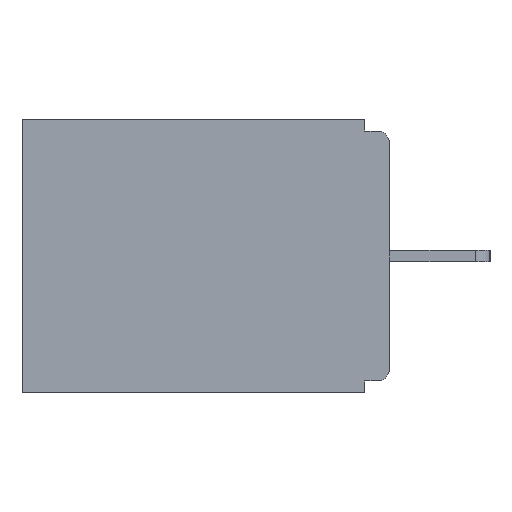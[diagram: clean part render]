
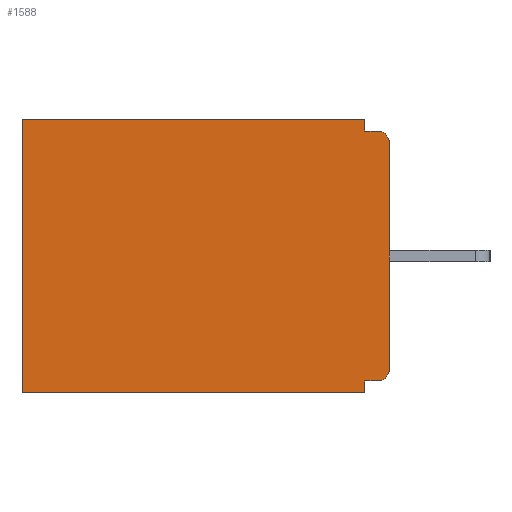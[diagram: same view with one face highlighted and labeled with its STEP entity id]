
A CAD part, left-side view. The second image highlights one B-rep face of the part: STEP entity #1588.
In plain terms, the highlighted planar face has unit normal (-1, 0, 0).
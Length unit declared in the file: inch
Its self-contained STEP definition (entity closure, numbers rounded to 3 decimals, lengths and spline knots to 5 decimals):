
#13 = VERTEX_POINT ( 'NONE', #4970 ) ;
#422 = CARTESIAN_POINT ( 'NONE',  ( 0.298, 0.031, -0.015 ) ) ;
#600 = CARTESIAN_POINT ( 'NONE',  ( 0.298, 0.015, -0.03 ) ) ;
#796 = LINE ( 'NONE', #12673, #15736 ) ;
#1186 = ORIENTED_EDGE ( 'NONE', *, *, #9808, .F. ) ;
#1255 = VECTOR ( 'NONE', #13989, 39.37008 ) ;
#1539 = EDGE_CURVE ( 'NONE', #2392, #10683, #5908, .T. ) ;
#1588 = ADVANCED_FACE ( 'NONE', ( #13958 ), #13664, .F. ) ;
#1697 = VECTOR ( 'NONE', #10648, 39.37008 ) ;
#1818 = CARTESIAN_POINT ( 'NONE',  ( 0.298, 0.46, 0. ) ) ;
#1954 = VECTOR ( 'NONE', #9693, 39.37008 ) ;
#2392 = VERTEX_POINT ( 'NONE', #10952 ) ;
#2653 = LINE ( 'NONE', #12521, #1954 ) ;
#2800 = LINE ( 'NONE', #5910, #7103 ) ;
#2859 = VERTEX_POINT ( 'NONE', #9610 ) ;
#3008 = CARTESIAN_POINT ( 'NONE',  ( 0.298, 0.031, -0.343 ) ) ;
#3226 = ORIENTED_EDGE ( 'NONE', *, *, #16742, .T. ) ;
#3445 = CARTESIAN_POINT ( 'NONE',  ( 0.298, 0., 0. ) ) ;
#3633 = DIRECTION ( 'NONE',  ( 1., 0., 0. ) ) ;
#3678 = EDGE_CURVE ( 'NONE', #2859, #18352, #16409, .T. ) ;
#3740 = EDGE_CURVE ( 'NONE', #10683, #18352, #2653, .T. ) ;
#4431 = ORIENTED_EDGE ( 'NONE', *, *, #3740, .F. ) ;
#4865 = CARTESIAN_POINT ( 'NONE',  ( 0.298, 0., -0.015 ) ) ;
#4866 = DIRECTION ( 'NONE',  ( 0., 0., -1. ) ) ;
#4970 = CARTESIAN_POINT ( 'NONE',  ( 0.298, 0., -0.03 ) ) ;
#4979 = DIRECTION ( 'NONE',  ( 0., 0., -1. ) ) ;
#5305 = VERTEX_POINT ( 'NONE', #6427 ) ;
#5325 = EDGE_CURVE ( 'NONE', #14812, #2859, #10608, .T. ) ;
#5695 = VERTEX_POINT ( 'NONE', #422 ) ;
#5908 = LINE ( 'NONE', #7524, #10994 ) ;
#5910 = CARTESIAN_POINT ( 'NONE',  ( 0.298, 0., -0.328 ) ) ;
#5939 = EDGE_CURVE ( 'NONE', #14812, #5695, #796, .T. ) ;
#6337 = DIRECTION ( 'NONE',  ( 0., 1., 0. ) ) ;
#6427 = CARTESIAN_POINT ( 'NONE',  ( 0.298, 0., -0.313 ) ) ;
#6455 = CARTESIAN_POINT ( 'NONE',  ( 0.298, 0.015, -0.015 ) ) ;
#6488 = VECTOR ( 'NONE', #14982, 39.37008 ) ;
#6786 = ORIENTED_EDGE ( 'NONE', *, *, #11349, .F. ) ;
#7095 = CARTESIAN_POINT ( 'NONE',  ( 0.298, 0.031, 0. ) ) ;
#7103 = VECTOR ( 'NONE', #14356, 39.37008 ) ;
#7524 = CARTESIAN_POINT ( 'NONE',  ( 0.298, 0.031, -0.343 ) ) ;
#7583 = ORIENTED_EDGE ( 'NONE', *, *, #3678, .T. ) ;
#7736 = DIRECTION ( 'NONE',  ( -1., 0., 0. ) ) ;
#7809 = LINE ( 'NONE', #4865, #1697 ) ;
#8090 = DIRECTION ( 'NONE',  ( 0., 0., -1. ) ) ;
#8124 = LINE ( 'NONE', #17129, #1255 ) ;
#9147 = DIRECTION ( 'NONE',  ( -1., 0., 0. ) ) ;
#9610 = CARTESIAN_POINT ( 'NONE',  ( 0.298, 0.46, 0. ) ) ;
#9693 = DIRECTION ( 'NONE',  ( 0., 1., 0. ) ) ;
#9808 = EDGE_CURVE ( 'NONE', #14503, #2392, #2800, .T. ) ;
#10076 = ORIENTED_EDGE ( 'NONE', *, *, #18541, .T. ) ;
#10523 = ORIENTED_EDGE ( 'NONE', *, *, #1539, .F. ) ;
#10608 = LINE ( 'NONE', #16571, #11460 ) ;
#10648 = DIRECTION ( 'NONE',  ( 0., -1., 0. ) ) ;
#10683 = VERTEX_POINT ( 'NONE', #3008 ) ;
#10952 = CARTESIAN_POINT ( 'NONE',  ( 0.298, 0.031, -0.328 ) ) ;
#10994 = VECTOR ( 'NONE', #13199, 39.37008 ) ;
#11256 = CIRCLE ( 'NONE', #14876, 0.015 ) ;
#11349 = EDGE_CURVE ( 'NONE', #5695, #14223, #7809, .T. ) ;
#11460 = VECTOR ( 'NONE', #6337, 39.37008 ) ;
#12340 = ORIENTED_EDGE ( 'NONE', *, *, #5939, .F. ) ;
#12401 = CIRCLE ( 'NONE', #16035, 0.015 ) ;
#12521 = CARTESIAN_POINT ( 'NONE',  ( 0.298, 0., -0.343 ) ) ;
#12673 = CARTESIAN_POINT ( 'NONE',  ( 0.298, 0.031, -0.343 ) ) ;
#13199 = DIRECTION ( 'NONE',  ( 0., 0., -1. ) ) ;
#13627 = EDGE_LOOP ( 'NONE', ( #3226, #6786, #12340, #14045, #7583, #4431, #10523, #1186, #10076, #16776 ) ) ;
#13664 = PLANE ( 'NONE',  #14324 ) ;
#13958 = FACE_OUTER_BOUND ( 'NONE', #13627, .T. ) ;
#13989 = DIRECTION ( 'NONE',  ( 0., 0., -1. ) ) ;
#14045 = ORIENTED_EDGE ( 'NONE', *, *, #5325, .T. ) ;
#14223 = VERTEX_POINT ( 'NONE', #6455 ) ;
#14324 = AXIS2_PLACEMENT_3D ( 'NONE', #3445, #3633, #8090 ) ;
#14356 = DIRECTION ( 'NONE',  ( 0., 1., 0. ) ) ;
#14503 = VERTEX_POINT ( 'NONE', #16016 ) ;
#14812 = VERTEX_POINT ( 'NONE', #7095 ) ;
#14876 = AXIS2_PLACEMENT_3D ( 'NONE', #18052, #9147, #4866 ) ;
#14982 = DIRECTION ( 'NONE',  ( 0., 0., -1. ) ) ;
#15736 = VECTOR ( 'NONE', #18466, 39.37008 ) ;
#16016 = CARTESIAN_POINT ( 'NONE',  ( 0.298, 0.015, -0.328 ) ) ;
#16035 = AXIS2_PLACEMENT_3D ( 'NONE', #600, #7736, #4979 ) ;
#16409 = LINE ( 'NONE', #1818, #6488 ) ;
#16571 = CARTESIAN_POINT ( 'NONE',  ( 0.298, 0., 0. ) ) ;
#16742 = EDGE_CURVE ( 'NONE', #13, #14223, #12401, .T. ) ;
#16776 = ORIENTED_EDGE ( 'NONE', *, *, #18282, .F. ) ;
#17129 = CARTESIAN_POINT ( 'NONE',  ( 0.298, 0., 0. ) ) ;
#17405 = CARTESIAN_POINT ( 'NONE',  ( 0.298, 0.46, -0.343 ) ) ;
#18052 = CARTESIAN_POINT ( 'NONE',  ( 0.298, 0.015, -0.313 ) ) ;
#18282 = EDGE_CURVE ( 'NONE', #13, #5305, #8124, .T. ) ;
#18352 = VERTEX_POINT ( 'NONE', #17405 ) ;
#18466 = DIRECTION ( 'NONE',  ( 0., 0., -1. ) ) ;
#18541 = EDGE_CURVE ( 'NONE', #14503, #5305, #11256, .T. ) ;
